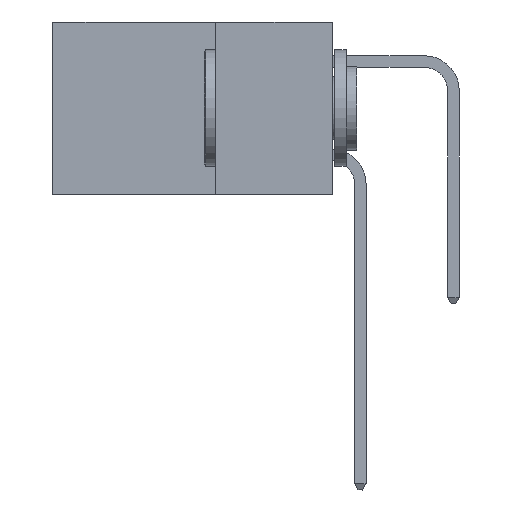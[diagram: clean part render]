
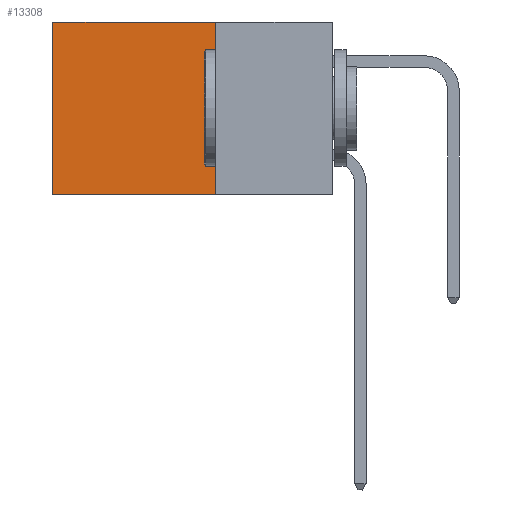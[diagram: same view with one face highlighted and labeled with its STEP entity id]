
A CAD part, left-side view. The second image highlights one B-rep face of the part: STEP entity #13308.
In plain terms, the highlighted planar face has unit normal (-1, 0, 0).
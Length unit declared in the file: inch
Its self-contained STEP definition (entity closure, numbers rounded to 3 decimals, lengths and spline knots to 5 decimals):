
#332 = VERTEX_POINT ( 'NONE', #6596 ) ;
#1346 = CARTESIAN_POINT ( 'NONE',  ( 0.298, 0.25, -0.37 ) ) ;
#3029 = EDGE_CURVE ( 'NONE', #4310, #29147, #6205, .T. ) ;
#4310 = VERTEX_POINT ( 'NONE', #15115 ) ;
#4572 = EDGE_CURVE ( 'NONE', #23863, #332, #6431, .T. ) ;
#6205 = LINE ( 'NONE', #26895, #12478 ) ;
#6431 = LINE ( 'NONE', #1346, #18003 ) ;
#6596 = CARTESIAN_POINT ( 'NONE',  ( 0.298, 0.6, -0.37 ) ) ;
#7447 = CARTESIAN_POINT ( 'NONE',  ( 0.298, 0.25, 0. ) ) ;
#7877 = DIRECTION ( 'NONE',  ( 1., 0., 0. ) ) ;
#8355 = CARTESIAN_POINT ( 'NONE',  ( 0.298, 0.6, 0. ) ) ;
#8366 = ORIENTED_EDGE ( 'NONE', *, *, #21330, .T. ) ;
#9472 = EDGE_LOOP ( 'NONE', ( #8366, #15669, #11306, #28298 ) ) ;
#9630 = AXIS2_PLACEMENT_3D ( 'NONE', #21639, #7877, #23924 ) ;
#11306 = ORIENTED_EDGE ( 'NONE', *, *, #19109, .F. ) ;
#12478 = VECTOR ( 'NONE', #27868, 39.37008 ) ;
#13266 = LINE ( 'NONE', #7447, #18607 ) ;
#13308 = ADVANCED_FACE ( 'NONE', ( #16135 ), #23831, .F. ) ;
#15115 = CARTESIAN_POINT ( 'NONE',  ( 0.298, 0.25, 0. ) ) ;
#15669 = ORIENTED_EDGE ( 'NONE', *, *, #4572, .F. ) ;
#15767 = CARTESIAN_POINT ( 'NONE',  ( 0.298, 0.25, -0.37 ) ) ;
#16135 = FACE_OUTER_BOUND ( 'NONE', #9472, .T. ) ;
#18003 = VECTOR ( 'NONE', #27645, 39.37008 ) ;
#18607 = VECTOR ( 'NONE', #18913, 39.37008 ) ;
#18862 = VECTOR ( 'NONE', #19801, 39.37008 ) ;
#18913 = DIRECTION ( 'NONE',  ( 0., 0., -1. ) ) ;
#19109 = EDGE_CURVE ( 'NONE', #4310, #23863, #13266, .T. ) ;
#19801 = DIRECTION ( 'NONE',  ( 0., 0., -1. ) ) ;
#21330 = EDGE_CURVE ( 'NONE', #29147, #332, #24921, .T. ) ;
#21639 = CARTESIAN_POINT ( 'NONE',  ( 0.298, 0.25, 0. ) ) ;
#23315 = CARTESIAN_POINT ( 'NONE',  ( 0.298, 0.6, 0. ) ) ;
#23831 = PLANE ( 'NONE',  #9630 ) ;
#23863 = VERTEX_POINT ( 'NONE', #15767 ) ;
#23924 = DIRECTION ( 'NONE',  ( 0., 0., -1. ) ) ;
#24921 = LINE ( 'NONE', #8355, #18862 ) ;
#26895 = CARTESIAN_POINT ( 'NONE',  ( 0.298, 0.25, 0. ) ) ;
#27645 = DIRECTION ( 'NONE',  ( 0., 1., 0. ) ) ;
#27868 = DIRECTION ( 'NONE',  ( 0., 1., 0. ) ) ;
#28298 = ORIENTED_EDGE ( 'NONE', *, *, #3029, .T. ) ;
#29147 = VERTEX_POINT ( 'NONE', #23315 ) ;
